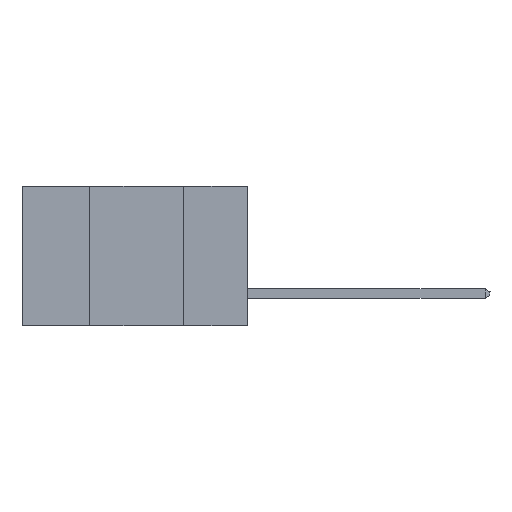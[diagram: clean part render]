
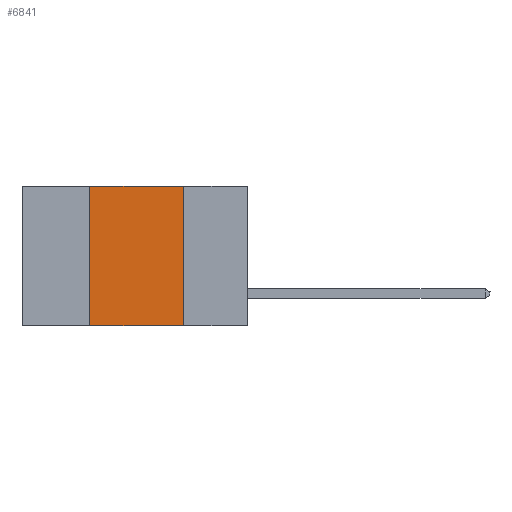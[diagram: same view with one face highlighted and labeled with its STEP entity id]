
A CAD part, left-side view. The second image highlights one B-rep face of the part: STEP entity #6841.
In plain terms, the highlighted planar face has unit normal (-1, 0, 0).
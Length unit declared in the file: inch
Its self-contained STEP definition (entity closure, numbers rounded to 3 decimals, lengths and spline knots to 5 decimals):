
#257 = EDGE_CURVE ( 'NONE', #13443, #15132, #4451, .T. ) ;
#2159 = CARTESIAN_POINT ( 'NONE',  ( 0., 0.6, -0.37 ) ) ;
#2529 = AXIS2_PLACEMENT_3D ( 'NONE', #13389, #9918, #3722 ) ;
#2677 = VECTOR ( 'NONE', #11438, 39.37008 ) ;
#3277 = DIRECTION ( 'NONE',  ( 0., 0., 1. ) ) ;
#3722 = DIRECTION ( 'NONE',  ( 0., 0., -1. ) ) ;
#4160 = CARTESIAN_POINT ( 'NONE',  ( 0., 0.17, -0.37 ) ) ;
#4326 = ORIENTED_EDGE ( 'NONE', *, *, #4942, .T. ) ;
#4451 = LINE ( 'NONE', #6781, #4821 ) ;
#4821 = VECTOR ( 'NONE', #3277, 39.37008 ) ;
#4942 = EDGE_CURVE ( 'NONE', #13443, #10098, #7827, .T. ) ;
#5052 = EDGE_CURVE ( 'NONE', #15132, #12289, #10138, .T. ) ;
#5995 = CARTESIAN_POINT ( 'NONE',  ( 0., 0.42, 0. ) ) ;
#6552 = EDGE_LOOP ( 'NONE', ( #7731, #12192, #8253, #4326 ) ) ;
#6781 = CARTESIAN_POINT ( 'NONE',  ( 0., 0.42, -0.37 ) ) ;
#6841 = ADVANCED_FACE ( 'NONE', ( #7379 ), #14455, .F. ) ;
#7379 = FACE_OUTER_BOUND ( 'NONE', #6552, .T. ) ;
#7731 = ORIENTED_EDGE ( 'NONE', *, *, #13023, .F. ) ;
#7827 = LINE ( 'NONE', #2159, #14545 ) ;
#8253 = ORIENTED_EDGE ( 'NONE', *, *, #257, .F. ) ;
#9079 = CARTESIAN_POINT ( 'NONE',  ( 0., 0.17, 0. ) ) ;
#9918 = DIRECTION ( 'NONE',  ( 1., 0., 0. ) ) ;
#10098 = VERTEX_POINT ( 'NONE', #14668 ) ;
#10138 = LINE ( 'NONE', #13747, #14454 ) ;
#10291 = DIRECTION ( 'NONE',  ( 0., -1., 0. ) ) ;
#11438 = DIRECTION ( 'NONE',  ( 0., 0., -1. ) ) ;
#12192 = ORIENTED_EDGE ( 'NONE', *, *, #5052, .F. ) ;
#12289 = VERTEX_POINT ( 'NONE', #9079 ) ;
#13023 = EDGE_CURVE ( 'NONE', #12289, #10098, #14720, .T. ) ;
#13389 = CARTESIAN_POINT ( 'NONE',  ( 0., 0.6, 0. ) ) ;
#13443 = VERTEX_POINT ( 'NONE', #13716 ) ;
#13716 = CARTESIAN_POINT ( 'NONE',  ( 0., 0.42, -0.37 ) ) ;
#13747 = CARTESIAN_POINT ( 'NONE',  ( 0., 0.6, 0. ) ) ;
#13821 = DIRECTION ( 'NONE',  ( 0., -1., 0. ) ) ;
#14454 = VECTOR ( 'NONE', #10291, 39.37008 ) ;
#14455 = PLANE ( 'NONE',  #2529 ) ;
#14545 = VECTOR ( 'NONE', #13821, 39.37008 ) ;
#14668 = CARTESIAN_POINT ( 'NONE',  ( 0., 0.17, -0.37 ) ) ;
#14720 = LINE ( 'NONE', #4160, #2677 ) ;
#15132 = VERTEX_POINT ( 'NONE', #5995 ) ;
